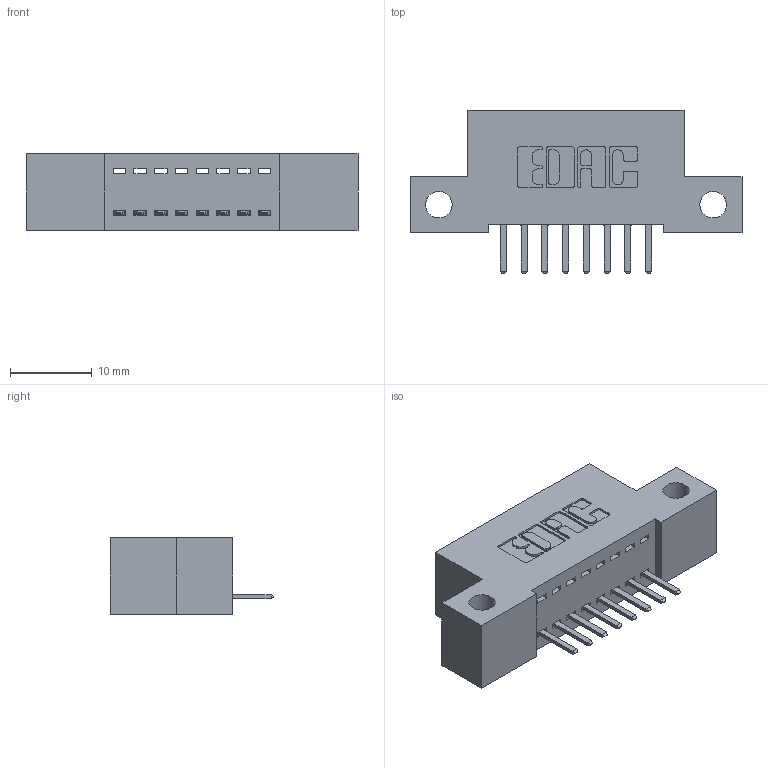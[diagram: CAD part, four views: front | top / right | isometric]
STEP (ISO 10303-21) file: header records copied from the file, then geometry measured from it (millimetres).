
FILE_DESCRIPTION (( 'STEP AP203' ), '1' );
FILE_NAME ('392-008-520-112.STEP', '2019-10-04T23:44:10', ( '' ), ( '' ), 'SwSTEP 2.0', 'SolidWorks 2016', '' );
FILE_SCHEMA (( 'CONFIG_CONTROL_DESIGN' ));
Length unit declared in the file: inch
Products named in the file (3): 342 Part_Side Mount; 345-292-001_345-293-120; 392-008-520-112
Assembly tree (9 placements, depth 2):
  392-008-520-112
    342 Part_Side Mount
    345-292-001_345-293-120  x8
Bounding box: 40.64 x 20.02 x 9.4 mm (x, y, z)
Volume: 3341.1 mm3; surface area: 4034.8 mm2
Topology: 9 solids, 9 shells, 606 faces, 1771 edges, 1158 vertices
Faces by surface type: plane 418, cylinder 188
Entity records: 9273 total; most frequent: CARTESIAN_POINT 1622, ORIENTED_EDGE 1554, DIRECTION 1425, EDGE_CURVE 777, VECTOR 645, LINE 645, VERTEX_POINT 514, AXIS2_PLACEMENT_3D 390
